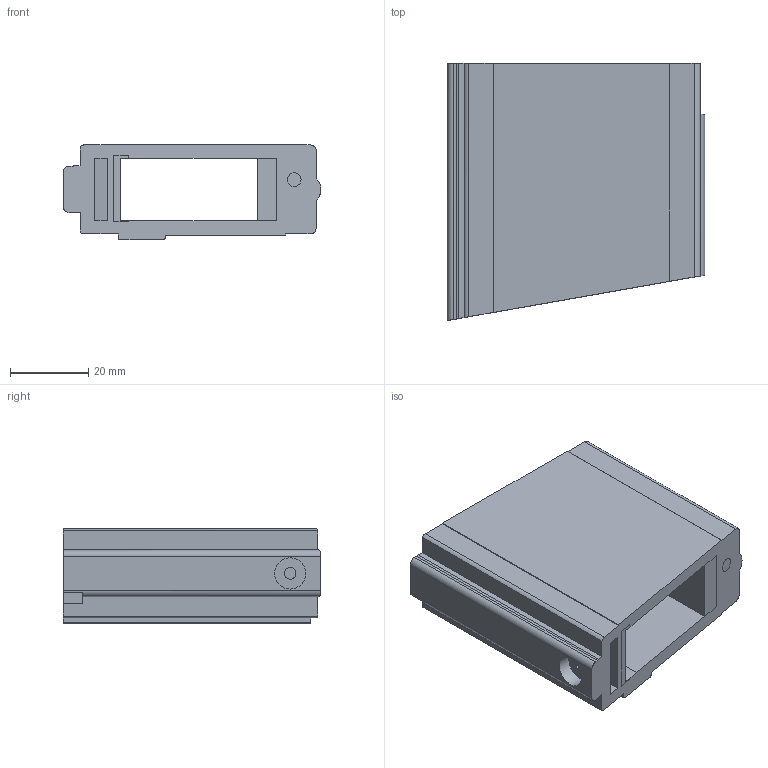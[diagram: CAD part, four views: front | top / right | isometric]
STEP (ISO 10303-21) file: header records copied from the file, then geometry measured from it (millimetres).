
FILE_DESCRIPTION(('FreeCAD Model'),'2;1');
FILE_NAME('Mag_Adapter.step', '2016-04-03T13:24:35',('Author'),(''), 'Open CASCADE STEP processor 6.8','FreeCAD','Unknown');
FILE_SCHEMA(('AUTOMOTIVE_DESIGN_CC2 { 1 2 10303 214 -1 1 5 4 }'));
Length unit declared in the file: millimetre
Products named in the file (1): Pocket015
Bounding box: 66.04 x 65.87 x 24.55 mm (x, y, z)
Volume: 51064.3 mm3; surface area: 19341.1 mm2
Topology: 1 solids, 1 shells, 64 faces, 192 edges, 133 vertices
Faces by surface type: plane 51, cylinder 13
Full cylindrical faces by diameter (mm): 3 x2, 8 x1
Entity records: 5169 total; most frequent: CARTESIAN_POINT 1642, DIRECTION 550, ORIENTED_EDGE 384, PCURVE 384, DEFINITIONAL_REPRESENTATION 384, LINE 365, VECTOR 365, EDGE_CURVE 192
